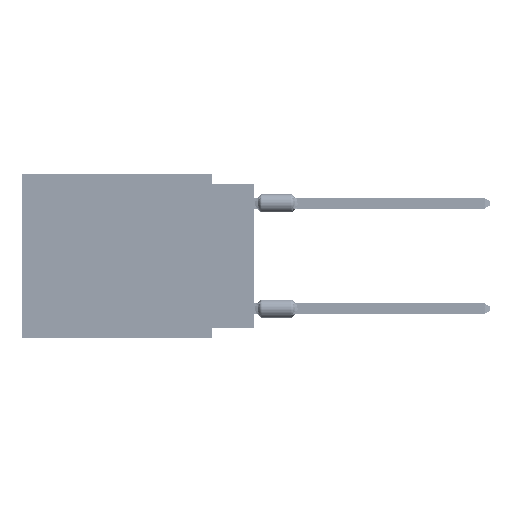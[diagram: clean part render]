
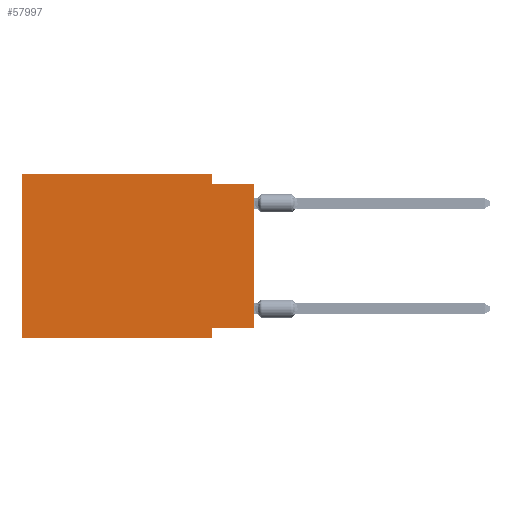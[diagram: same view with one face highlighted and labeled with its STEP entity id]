
A CAD part, left-side view. The second image highlights one B-rep face of the part: STEP entity #57997.
In plain terms, the highlighted planar face has unit normal (-1, 0, 0).
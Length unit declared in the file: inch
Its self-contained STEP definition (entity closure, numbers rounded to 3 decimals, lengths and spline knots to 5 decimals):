
#283 = VECTOR ( 'NONE', #26673, 39.37008 ) ;
#859 = EDGE_CURVE ( 'NONE', #39341, #72216, #89059, .T. ) ;
#864 = LINE ( 'NONE', #83788, #28240 ) ;
#1391 = ORIENTED_EDGE ( 'NONE', *, *, #83192, .F. ) ;
#3426 = CARTESIAN_POINT ( 'NONE',  ( 0., 0.55, 0. ) ) ;
#4935 = EDGE_CURVE ( 'NONE', #70651, #21045, #7163, .T. ) ;
#5853 = DIRECTION ( 'NONE',  ( 0., -1., 0. ) ) ;
#6812 = DIRECTION ( 'NONE',  ( 0., 0., -1. ) ) ;
#7163 = LINE ( 'NONE', #34996, #37007 ) ;
#11710 = CARTESIAN_POINT ( 'NONE',  ( 0., 0.1, -0.025 ) ) ;
#14324 = DIRECTION ( 'NONE',  ( 0., 0., -1. ) ) ;
#15368 = DIRECTION ( 'NONE',  ( 0., 0., 1. ) ) ;
#15576 = CARTESIAN_POINT ( 'NONE',  ( 0., 0.1, -0.39 ) ) ;
#15960 = VECTOR ( 'NONE', #58709, 39.37008 ) ;
#16287 = CARTESIAN_POINT ( 'NONE',  ( 0., 0.55, 0. ) ) ;
#19666 = DIRECTION ( 'NONE',  ( 0., -1., 0. ) ) ;
#19817 = PLANE ( 'NONE',  #37102 ) ;
#20747 = VERTEX_POINT ( 'NONE', #11710 ) ;
#21045 = VERTEX_POINT ( 'NONE', #28991 ) ;
#21993 = ORIENTED_EDGE ( 'NONE', *, *, #26052, .F. ) ;
#22146 = CARTESIAN_POINT ( 'NONE',  ( 0., 0., -0.365 ) ) ;
#24861 = ORIENTED_EDGE ( 'NONE', *, *, #859, .F. ) ;
#24862 = VECTOR ( 'NONE', #39880, 39.37008 ) ;
#25301 = LINE ( 'NONE', #3426, #24862 ) ;
#26052 = EDGE_CURVE ( 'NONE', #40608, #67364, #41914, .T. ) ;
#26673 = DIRECTION ( 'NONE',  ( 0., -1., 0. ) ) ;
#27114 = FACE_OUTER_BOUND ( 'NONE', #84992, .T. ) ;
#27345 = CARTESIAN_POINT ( 'NONE',  ( 0., 0.1, -0.39 ) ) ;
#27368 = ORIENTED_EDGE ( 'NONE', *, *, #32289, .F. ) ;
#28240 = VECTOR ( 'NONE', #77397, 39.37008 ) ;
#28294 = CARTESIAN_POINT ( 'NONE',  ( 0., 0.1, 0. ) ) ;
#28991 = CARTESIAN_POINT ( 'NONE',  ( 0., 0., -0.025 ) ) ;
#30320 = VECTOR ( 'NONE', #6812, 39.37008 ) ;
#32289 = EDGE_CURVE ( 'NONE', #20747, #21045, #32464, .T. ) ;
#32464 = LINE ( 'NONE', #61994, #58412 ) ;
#34996 = CARTESIAN_POINT ( 'NONE',  ( 0., 0., 0. ) ) ;
#37007 = VECTOR ( 'NONE', #15368, 39.37008 ) ;
#37102 = AXIS2_PLACEMENT_3D ( 'NONE', #70347, #83566, #14324 ) ;
#39341 = VERTEX_POINT ( 'NONE', #16287 ) ;
#39880 = DIRECTION ( 'NONE',  ( 0., 0., 1. ) ) ;
#40608 = VERTEX_POINT ( 'NONE', #55096 ) ;
#41914 = LINE ( 'NONE', #27345, #30320 ) ;
#50902 = ORIENTED_EDGE ( 'NONE', *, *, #72536, .T. ) ;
#52459 = ORIENTED_EDGE ( 'NONE', *, *, #4935, .T. ) ;
#54887 = CARTESIAN_POINT ( 'NONE',  ( 0., 0.55, 0. ) ) ;
#55096 = CARTESIAN_POINT ( 'NONE',  ( 0., 0.1, -0.365 ) ) ;
#57262 = EDGE_CURVE ( 'NONE', #72216, #20747, #864, .T. ) ;
#57997 = ADVANCED_FACE ( 'NONE', ( #27114 ), #19817, .F. ) ;
#58258 = CARTESIAN_POINT ( 'NONE',  ( 0., 0., -0.365 ) ) ;
#58412 = VECTOR ( 'NONE', #19666, 39.37008 ) ;
#58709 = DIRECTION ( 'NONE',  ( 0., 1., 0. ) ) ;
#61934 = CARTESIAN_POINT ( 'NONE',  ( 0., 0.55, -0.39 ) ) ;
#61994 = CARTESIAN_POINT ( 'NONE',  ( 0., 0., -0.025 ) ) ;
#62281 = EDGE_CURVE ( 'NONE', #70651, #40608, #79682, .T. ) ;
#67364 = VERTEX_POINT ( 'NONE', #15576 ) ;
#69957 = CARTESIAN_POINT ( 'NONE',  ( 0., 0.55, -0.39 ) ) ;
#70347 = CARTESIAN_POINT ( 'NONE',  ( 0., 0.55, 0. ) ) ;
#70651 = VERTEX_POINT ( 'NONE', #22146 ) ;
#72216 = VERTEX_POINT ( 'NONE', #28294 ) ;
#72536 = EDGE_CURVE ( 'NONE', #81749, #67364, #81045, .T. ) ;
#77397 = DIRECTION ( 'NONE',  ( 0., 0., -1. ) ) ;
#77548 = VECTOR ( 'NONE', #5853, 39.37008 ) ;
#79682 = LINE ( 'NONE', #58258, #15960 ) ;
#81045 = LINE ( 'NONE', #61934, #77548 ) ;
#81749 = VERTEX_POINT ( 'NONE', #69957 ) ;
#83189 = ORIENTED_EDGE ( 'NONE', *, *, #62281, .F. ) ;
#83192 = EDGE_CURVE ( 'NONE', #81749, #39341, #25301, .T. ) ;
#83566 = DIRECTION ( 'NONE',  ( 1., 0., 0. ) ) ;
#83776 = ORIENTED_EDGE ( 'NONE', *, *, #57262, .F. ) ;
#83788 = CARTESIAN_POINT ( 'NONE',  ( 0., 0.1, 0. ) ) ;
#84992 = EDGE_LOOP ( 'NONE', ( #52459, #27368, #83776, #24861, #1391, #50902, #21993, #83189 ) ) ;
#89059 = LINE ( 'NONE', #54887, #283 ) ;
